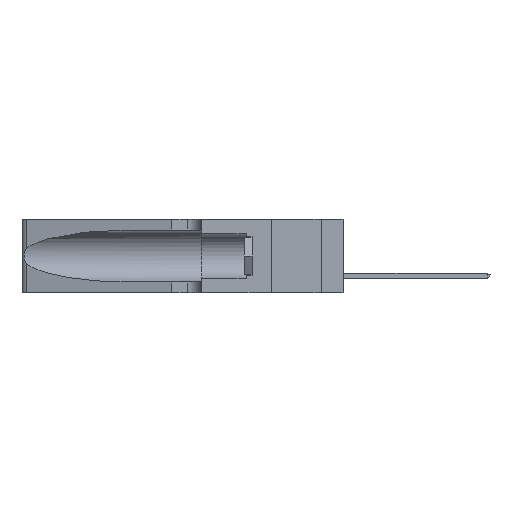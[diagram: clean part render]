
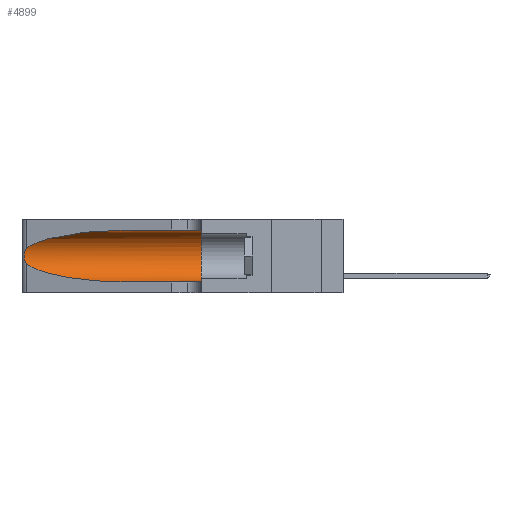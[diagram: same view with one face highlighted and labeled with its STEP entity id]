
A CAD part, left-side view. The second image highlights one B-rep face of the part: STEP entity #4899.
In plain terms, the highlighted cylindrical face has radius 3.308 mm (diameter 6.617 mm), a partial arc.
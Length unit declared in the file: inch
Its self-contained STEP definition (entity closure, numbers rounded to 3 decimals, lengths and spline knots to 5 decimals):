
#87 = CARTESIAN_POINT ( 'NONE',  ( 0.25639, 1.23186, 0.15144 ) ) ;
#1434 = EDGE_CURVE ( 'NONE', #3389, #7617, #4110, .T. ) ;
#1554 = CARTESIAN_POINT ( 'NONE',  ( 0.1305, 1.61858, 0.185 ) ) ;
#2170 = CARTESIAN_POINT ( 'NONE',  ( 0.25555, 1.22993, 0.14849 ) ) ;
#2311 = VERTEX_POINT ( 'NONE', #17271 ) ;
#2443 = EDGE_CURVE ( 'NONE', #25665, #3389, #19400, .T. ) ;
#3330 = CARTESIAN_POINT ( 'NONE',  ( 0.18966, 0.96281, 0.31525 ) ) ;
#3389 = VERTEX_POINT ( 'NONE', #12588 ) ;
#3692 = CARTESIAN_POINT ( 'NONE',  ( 0.1305, 0.72297, 0.31525 ) ) ;
#3830 = DIRECTION ( 'NONE',  ( 0., 0., -1. ) ) ;
#4110 =( BOUNDED_CURVE ( )  B_SPLINE_CURVE ( 3, ( #10716, #21047, #4733, #8646 ),
 .UNSPECIFIED., .F., .F. ) 
 B_SPLINE_CURVE_WITH_KNOTS ( ( 4, 4 ),
 ( 3.44316, 4.71239 ),
 .UNSPECIFIED. ) 
 CURVE ( )  GEOMETRIC_REPRESENTATION_ITEM ( )  RATIONAL_B_SPLINE_CURVE ( ( 1., 0.87, 0.87, 1. ) ) 
 REPRESENTATION_ITEM ( '' )  );
#4114 = ORIENTED_EDGE ( 'NONE', *, *, #11473, .T. ) ;
#4276 = EDGE_CURVE ( 'NONE', #22545, #6242, #4682, .T. ) ;
#4682 = LINE ( 'NONE', #5797, #8261 ) ;
#4733 = CARTESIAN_POINT ( 'NONE',  ( 0.18966, 0.96281, 0.05475 ) ) ;
#4899 = ADVANCED_FACE ( 'NONE', ( #7905 ), #10477, .F. ) ;
#5432 = CARTESIAN_POINT ( 'NONE',  ( 0.25487, 1.22718, 0.22369 ) ) ;
#5512 = CARTESIAN_POINT ( 'NONE',  ( 0.1305, 0.72297, 0.31525 ) ) ;
#5544 = DIRECTION ( 'NONE',  ( 0., -1., 0. ) ) ;
#5797 = CARTESIAN_POINT ( 'NONE',  ( 0.1305, 1.61858, 0.31525 ) ) ;
#6120 = VECTOR ( 'NONE', #12870, 39.37008 ) ;
#6242 = VERTEX_POINT ( 'NONE', #20993 ) ;
#7311 = CARTESIAN_POINT ( 'NONE',  ( 0.1305, 0.72297, 0.05475 ) ) ;
#7617 = VERTEX_POINT ( 'NONE', #7311 ) ;
#7905 = FACE_OUTER_BOUND ( 'NONE', #11375, .T. ) ;
#8261 = VECTOR ( 'NONE', #5544, 39.37008 ) ;
#8646 = CARTESIAN_POINT ( 'NONE',  ( 0.1305, 0.72297, 0.05475 ) ) ;
#9292 = CARTESIAN_POINT ( 'NONE',  ( 0.25787, 1.23484, 0.2124 ) ) ;
#9481 = CARTESIAN_POINT ( 'NONE',  ( 0.25487, 1.22718, 0.22369 ) ) ;
#9561 = CARTESIAN_POINT ( 'NONE',  ( 0.26075, 1.23896, 0.178 ) ) ;
#10477 = CYLINDRICAL_SURFACE ( 'NONE', #23252, 0.13025 ) ;
#10584 =( BOUNDED_CURVE ( )  B_SPLINE_CURVE ( 3, ( #5512, #3330, #26120, #5432 ),
 .UNSPECIFIED., .F., .F. ) 
 B_SPLINE_CURVE_WITH_KNOTS ( ( 4, 4 ),
 ( 1.5708, 2.84003 ),
 .UNSPECIFIED. ) 
 CURVE ( )  GEOMETRIC_REPRESENTATION_ITEM ( )  RATIONAL_B_SPLINE_CURVE ( ( 1., 0.87, 0.87, 1. ) ) 
 REPRESENTATION_ITEM ( '' )  );
#10716 = CARTESIAN_POINT ( 'NONE',  ( 0.25487, 1.22718, 0.14631 ) ) ;
#10777 = ORIENTED_EDGE ( 'NONE', *, *, #14974, .T. ) ;
#11359 = CARTESIAN_POINT ( 'NONE',  ( 0.25854, 1.2359, 0.20912 ) ) ;
#11375 = EDGE_LOOP ( 'NONE', ( #4114, #14527, #18883, #10777, #21958, #14711 ) ) ;
#11473 = EDGE_CURVE ( 'NONE', #22545, #25665, #10584, .T. ) ;
#11885 = CARTESIAN_POINT ( 'NONE',  ( 0.26017, 1.23833, 0.17102 ) ) ;
#12588 = CARTESIAN_POINT ( 'NONE',  ( 0.25487, 1.22718, 0.14631 ) ) ;
#12870 = DIRECTION ( 'NONE',  ( 0., -1., 0. ) ) ;
#13700 = CARTESIAN_POINT ( 'NONE',  ( 0.25789, 1.23486, 0.15765 ) ) ;
#14527 = ORIENTED_EDGE ( 'NONE', *, *, #2443, .T. ) ;
#14711 = ORIENTED_EDGE ( 'NONE', *, *, #4276, .F. ) ;
#14974 = EDGE_CURVE ( 'NONE', #7617, #2311, #18126, .T. ) ;
#15432 = CARTESIAN_POINT ( 'NONE',  ( 0.25555, 1.22994, 0.2215 ) ) ;
#16058 = CARTESIAN_POINT ( 'NONE',  ( 0.25856, 1.23593, 0.16098 ) ) ;
#16369 = EDGE_CURVE ( 'NONE', #6242, #2311, #17022, .T. ) ;
#17022 = CIRCLE ( 'NONE', #22616, 0.13025 ) ;
#17271 = CARTESIAN_POINT ( 'NONE',  ( 0.1305, 0.35, 0.05475 ) ) ;
#18100 = CARTESIAN_POINT ( 'NONE',  ( 0.25487, 1.22718, 0.22369 ) ) ;
#18126 = LINE ( 'NONE', #23242, #6120 ) ;
#18763 = CARTESIAN_POINT ( 'NONE',  ( 0.25487, 1.22718, 0.14631 ) ) ;
#18883 = ORIENTED_EDGE ( 'NONE', *, *, #1434, .T. ) ;
#19400 = B_SPLINE_CURVE_WITH_KNOTS ( 'NONE', 3,
 ( #9481, #15432, #19606, #9292, #11359, #24259, #20233, #9561, #11885, #16058, #13700, #87, #2170, #18763 ),
 .UNSPECIFIED., .F., .F.,
 ( 4, 2, 2, 2, 2, 2, 4 ),
 ( 0., 0.00027, 0.00053, 0.00107, 0.0016, 0.00187, 0.00214 ),
 .UNSPECIFIED. ) ;
#19606 = CARTESIAN_POINT ( 'NONE',  ( 0.25639, 1.23184, 0.21858 ) ) ;
#20148 = DIRECTION ( 'NONE',  ( 0., -1., 0. ) ) ;
#20233 = CARTESIAN_POINT ( 'NONE',  ( 0.26075, 1.23896, 0.19203 ) ) ;
#20386 = CARTESIAN_POINT ( 'NONE',  ( 0.1305, 0.35, 0.185 ) ) ;
#20466 = DIRECTION ( 'NONE',  ( 0., 0., 1. ) ) ;
#20993 = CARTESIAN_POINT ( 'NONE',  ( 0.1305, 0.35, 0.31525 ) ) ;
#21047 = CARTESIAN_POINT ( 'NONE',  ( 0.2373, 1.15595, 0.08982 ) ) ;
#21958 = ORIENTED_EDGE ( 'NONE', *, *, #16369, .F. ) ;
#22545 = VERTEX_POINT ( 'NONE', #3692 ) ;
#22616 = AXIS2_PLACEMENT_3D ( 'NONE', #20386, #24574, #20466 ) ;
#23242 = CARTESIAN_POINT ( 'NONE',  ( 0.1305, 1.61858, 0.05475 ) ) ;
#23252 = AXIS2_PLACEMENT_3D ( 'NONE', #1554, #20148, #3830 ) ;
#24259 = CARTESIAN_POINT ( 'NONE',  ( 0.26018, 1.23835, 0.19895 ) ) ;
#24574 = DIRECTION ( 'NONE',  ( 0., 1., 0. ) ) ;
#25665 = VERTEX_POINT ( 'NONE', #18100 ) ;
#26120 = CARTESIAN_POINT ( 'NONE',  ( 0.2373, 1.15595, 0.28018 ) ) ;
